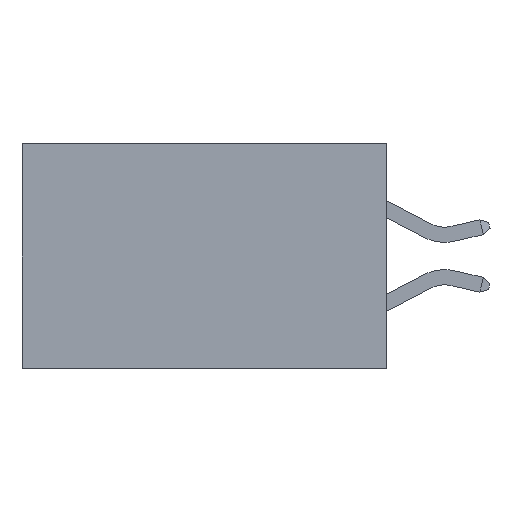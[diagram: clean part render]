
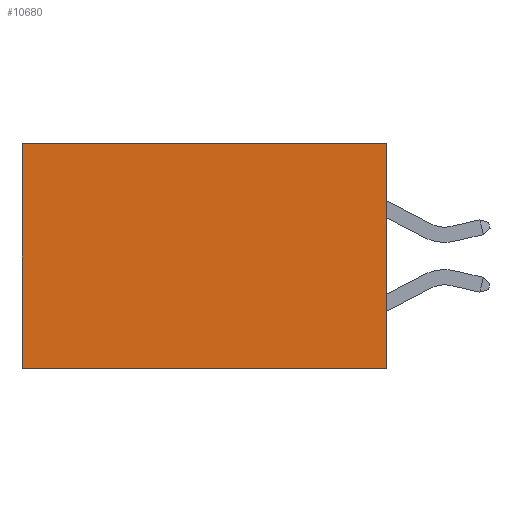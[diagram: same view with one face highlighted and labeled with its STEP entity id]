
A CAD part, left-side view. The second image highlights one B-rep face of the part: STEP entity #10680.
In plain terms, the highlighted planar face has unit normal (-1, 0, 0).
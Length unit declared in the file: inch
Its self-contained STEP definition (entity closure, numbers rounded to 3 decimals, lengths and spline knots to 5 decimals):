
#450 = CARTESIAN_POINT ( 'NONE',  ( 0.2615, 0., -0.37 ) ) ;
#1026 = VERTEX_POINT ( 'NONE', #6692 ) ;
#1209 = VECTOR ( 'NONE', #9916, 39.37008 ) ;
#1246 = CARTESIAN_POINT ( 'NONE',  ( 0.2615, 0., -0.37 ) ) ;
#1269 = ORIENTED_EDGE ( 'NONE', *, *, #10920, .F. ) ;
#1731 = LINE ( 'NONE', #6110, #4596 ) ;
#2447 = EDGE_CURVE ( 'NONE', #4996, #1026, #9925, .T. ) ;
#3646 = VERTEX_POINT ( 'NONE', #12382 ) ;
#4361 = CARTESIAN_POINT ( 'NONE',  ( 0.2615, 0., 0. ) ) ;
#4432 = CARTESIAN_POINT ( 'NONE',  ( 0.2615, 0., 0. ) ) ;
#4580 = EDGE_LOOP ( 'NONE', ( #6060, #6530, #1269, #4795 ) ) ;
#4596 = VECTOR ( 'NONE', #9406, 39.37008 ) ;
#4795 = ORIENTED_EDGE ( 'NONE', *, *, #2447, .T. ) ;
#4909 = LINE ( 'NONE', #450, #10977 ) ;
#4996 = VERTEX_POINT ( 'NONE', #4361 ) ;
#5588 = EDGE_CURVE ( 'NONE', #3646, #6514, #8709, .T. ) ;
#5750 = DIRECTION ( 'NONE',  ( 1., 0., 0. ) ) ;
#6060 = ORIENTED_EDGE ( 'NONE', *, *, #10984, .T. ) ;
#6110 = CARTESIAN_POINT ( 'NONE',  ( 0.2615, 0.6, -0.37 ) ) ;
#6316 = VECTOR ( 'NONE', #8790, 39.37008 ) ;
#6514 = VERTEX_POINT ( 'NONE', #6679 ) ;
#6530 = ORIENTED_EDGE ( 'NONE', *, *, #5588, .F. ) ;
#6679 = CARTESIAN_POINT ( 'NONE',  ( 0.2615, 0.6, -0.37 ) ) ;
#6692 = CARTESIAN_POINT ( 'NONE',  ( 0.2615, 0.6, 0. ) ) ;
#6761 = DIRECTION ( 'NONE',  ( 0., 0., -1. ) ) ;
#8114 = DIRECTION ( 'NONE',  ( 0., 0., -1. ) ) ;
#8691 = CARTESIAN_POINT ( 'NONE',  ( 0.2615, 0., -0.37 ) ) ;
#8709 = LINE ( 'NONE', #1246, #1209 ) ;
#8790 = DIRECTION ( 'NONE',  ( 0., 1., 0. ) ) ;
#9399 = AXIS2_PLACEMENT_3D ( 'NONE', #8691, #5750, #6761 ) ;
#9406 = DIRECTION ( 'NONE',  ( 0., 0., -1. ) ) ;
#9757 = FACE_OUTER_BOUND ( 'NONE', #4580, .T. ) ;
#9916 = DIRECTION ( 'NONE',  ( 0., 1., 0. ) ) ;
#9925 = LINE ( 'NONE', #4432, #6316 ) ;
#10680 = ADVANCED_FACE ( 'NONE', ( #9757 ), #14123, .F. ) ;
#10920 = EDGE_CURVE ( 'NONE', #4996, #3646, #4909, .T. ) ;
#10977 = VECTOR ( 'NONE', #8114, 39.37008 ) ;
#10984 = EDGE_CURVE ( 'NONE', #1026, #6514, #1731, .T. ) ;
#12382 = CARTESIAN_POINT ( 'NONE',  ( 0.2615, 0., -0.37 ) ) ;
#14123 = PLANE ( 'NONE',  #9399 ) ;
